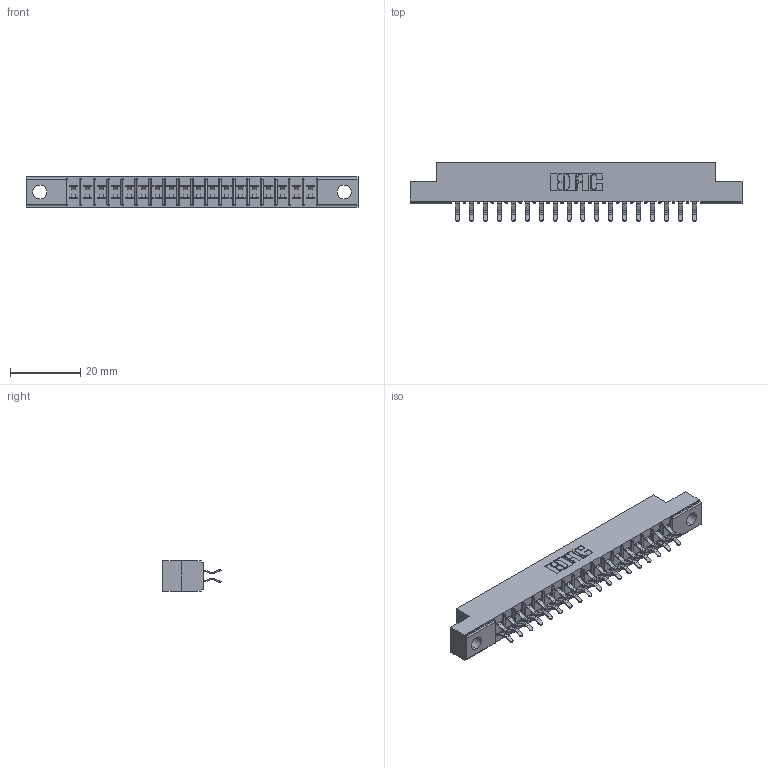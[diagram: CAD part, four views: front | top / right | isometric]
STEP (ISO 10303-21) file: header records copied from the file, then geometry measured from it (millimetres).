
FILE_DESCRIPTION (( 'STEP AP203' ), '1' );
FILE_NAME ('355-036-556-504.STEP', '2019-09-11T10:02:49', ( '' ), ( '' ), 'SwSTEP 2.0', 'SolidWorks 2016', '' );
FILE_SCHEMA (( 'CONFIG_CONTROL_DESIGN' ));
Length unit declared in the file: inch
Products named in the file (3): 305-290-001_556; 355-036-556-504; 305 Part_.156 Dia
Assembly tree (37 placements, depth 2):
  355-036-556-504
    305 Part_.156 Dia
    305-290-001_556  x36
Bounding box: 94.34 x 16.64 x 8.71 mm (x, y, z)
Volume: 5557.4 mm3; surface area: 10742.1 mm2
Topology: 37 solids, 37 shells, 2146 faces, 6166 edges, 4012 vertices
Faces by surface type: plane 1198, cylinder 876, sphere 72
Entity records: 23051 total; most frequent: CARTESIAN_POINT 3822, ORIENTED_EDGE 3788, DIRECTION 3712, EDGE_CURVE 1894, LINE 1508, VECTOR 1508, VERTEX_POINT 1212, AXIS2_PLACEMENT_3D 1102
